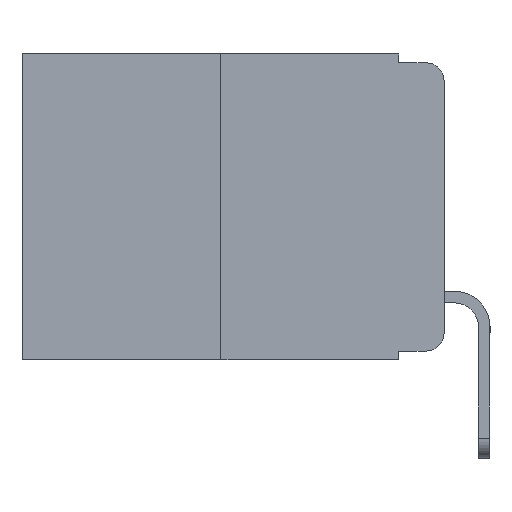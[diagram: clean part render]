
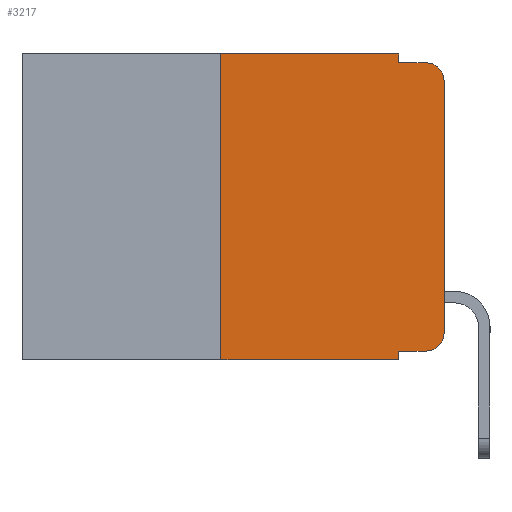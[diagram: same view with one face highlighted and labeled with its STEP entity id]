
A CAD part, left-side view. The second image highlights one B-rep face of the part: STEP entity #3217.
In plain terms, the highlighted planar face has unit normal (-1, 0, 0).
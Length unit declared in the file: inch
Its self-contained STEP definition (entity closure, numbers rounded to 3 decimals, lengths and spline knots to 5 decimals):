
#124 = DIRECTION ( 'NONE',  ( -1., 0., 0. ) ) ;
#164 = EDGE_CURVE ( 'NONE', #3692, #11621, #11876, .T. ) ;
#549 = PLANE ( 'NONE',  #6220 ) ;
#786 = ORIENTED_EDGE ( 'NONE', *, *, #994, .F. ) ;
#886 = EDGE_CURVE ( 'NONE', #7937, #5709, #5619, .T. ) ;
#915 = EDGE_CURVE ( 'NONE', #3985, #5709, #7725, .T. ) ;
#959 = EDGE_CURVE ( 'NONE', #8547, #3692, #6330, .T. ) ;
#992 = EDGE_CURVE ( 'NONE', #2459, #7937, #12639, .T. ) ;
#994 = EDGE_CURVE ( 'NONE', #11621, #3985, #9289, .T. ) ;
#1360 = ORIENTED_EDGE ( 'NONE', *, *, #164, .F. ) ;
#1522 = EDGE_CURVE ( 'NONE', #11440, #16614, #14480, .T. ) ;
#1541 = CARTESIAN_POINT ( 'NONE',  ( 0., 0.02, -0.01 ) ) ;
#2351 = CARTESIAN_POINT ( 'NONE',  ( 0., 0.25, -0.343 ) ) ;
#2446 = ORIENTED_EDGE ( 'NONE', *, *, #14874, .F. ) ;
#2459 = VERTEX_POINT ( 'NONE', #6976 ) ;
#2882 = CARTESIAN_POINT ( 'NONE',  ( 0., 0.051, -0.333 ) ) ;
#2959 = ORIENTED_EDGE ( 'NONE', *, *, #9412, .T. ) ;
#3060 = DIRECTION ( 'NONE',  ( 0., 0., -1. ) ) ;
#3217 = ADVANCED_FACE ( 'NONE', ( #4060 ), #549, .F. ) ;
#3358 = CARTESIAN_POINT ( 'NONE',  ( 0., 0.02, -0.313 ) ) ;
#3692 = VERTEX_POINT ( 'NONE', #15382 ) ;
#3832 = EDGE_CURVE ( 'NONE', #8547, #16906, #17649, .T. ) ;
#3947 = DIRECTION ( 'NONE',  ( 1., 0., 0. ) ) ;
#3985 = VERTEX_POINT ( 'NONE', #11628 ) ;
#4060 = FACE_OUTER_BOUND ( 'NONE', #10998, .T. ) ;
#4124 = AXIS2_PLACEMENT_3D ( 'NONE', #6033, #124, #3060 ) ;
#4198 = VECTOR ( 'NONE', #5405, 39.37008 ) ;
#4660 = ORIENTED_EDGE ( 'NONE', *, *, #915, .F. ) ;
#4742 = VECTOR ( 'NONE', #6989, 39.37008 ) ;
#4897 = DIRECTION ( 'NONE',  ( 0., 0., -1. ) ) ;
#5322 = CARTESIAN_POINT ( 'NONE',  ( 0., 0.051, -0.01 ) ) ;
#5331 = VECTOR ( 'NONE', #10508, 39.37008 ) ;
#5405 = DIRECTION ( 'NONE',  ( 0., -1., 0. ) ) ;
#5424 = CARTESIAN_POINT ( 'NONE',  ( 0., 0., 0. ) ) ;
#5515 = DIRECTION ( 'NONE',  ( 0., 0., 1. ) ) ;
#5593 = ORIENTED_EDGE ( 'NONE', *, *, #959, .F. ) ;
#5619 = CIRCLE ( 'NONE', #4124, 0.02 ) ;
#5709 = VERTEX_POINT ( 'NONE', #1541 ) ;
#6033 = CARTESIAN_POINT ( 'NONE',  ( 0., 0.02, -0.03 ) ) ;
#6220 = AXIS2_PLACEMENT_3D ( 'NONE', #15824, #3947, #13518 ) ;
#6330 = LINE ( 'NONE', #8835, #7257 ) ;
#6976 = CARTESIAN_POINT ( 'NONE',  ( 0., 0., -0.313 ) ) ;
#6989 = DIRECTION ( 'NONE',  ( 0., -1., 0. ) ) ;
#7189 = AXIS2_PLACEMENT_3D ( 'NONE', #3358, #13056, #4897 ) ;
#7226 = VECTOR ( 'NONE', #15899, 39.37008 ) ;
#7257 = VECTOR ( 'NONE', #9005, 39.37008 ) ;
#7295 = CARTESIAN_POINT ( 'NONE',  ( 0., 0.051, -0.333 ) ) ;
#7679 = DIRECTION ( 'NONE',  ( 0., 0., -1. ) ) ;
#7725 = LINE ( 'NONE', #5322, #4198 ) ;
#7937 = VERTEX_POINT ( 'NONE', #15793 ) ;
#8032 = CIRCLE ( 'NONE', #7189, 0.02 ) ;
#8547 = VERTEX_POINT ( 'NONE', #2351 ) ;
#8835 = CARTESIAN_POINT ( 'NONE',  ( 0., 0.25, 0. ) ) ;
#9005 = DIRECTION ( 'NONE',  ( 0., 0., 1. ) ) ;
#9289 = LINE ( 'NONE', #15626, #15413 ) ;
#9412 = EDGE_CURVE ( 'NONE', #16614, #2459, #8032, .T. ) ;
#10404 = CARTESIAN_POINT ( 'NONE',  ( 0., 0.051, 0. ) ) ;
#10508 = DIRECTION ( 'NONE',  ( 0., -1., 0. ) ) ;
#10998 = EDGE_LOOP ( 'NONE', ( #11306, #11693, #4660, #786, #1360, #5593, #16322, #2446, #13564, #2959 ) ) ;
#11306 = ORIENTED_EDGE ( 'NONE', *, *, #992, .T. ) ;
#11440 = VERTEX_POINT ( 'NONE', #2882 ) ;
#11621 = VERTEX_POINT ( 'NONE', #10404 ) ;
#11628 = CARTESIAN_POINT ( 'NONE',  ( 0., 0.051, -0.01 ) ) ;
#11693 = ORIENTED_EDGE ( 'NONE', *, *, #886, .T. ) ;
#11854 = LINE ( 'NONE', #15244, #17735 ) ;
#11876 = LINE ( 'NONE', #14030, #5331 ) ;
#12639 = LINE ( 'NONE', #5424, #13376 ) ;
#13056 = DIRECTION ( 'NONE',  ( -1., 0., 0. ) ) ;
#13376 = VECTOR ( 'NONE', #5515, 39.37008 ) ;
#13446 = CARTESIAN_POINT ( 'NONE',  ( 0., 0.02, -0.333 ) ) ;
#13518 = DIRECTION ( 'NONE',  ( 0., 0., -1. ) ) ;
#13564 = ORIENTED_EDGE ( 'NONE', *, *, #1522, .T. ) ;
#14030 = CARTESIAN_POINT ( 'NONE',  ( 0., 0.473, 0. ) ) ;
#14480 = LINE ( 'NONE', #7295, #7226 ) ;
#14631 = DIRECTION ( 'NONE',  ( 0., 0., -1. ) ) ;
#14704 = CARTESIAN_POINT ( 'NONE',  ( 0., 0.473, -0.343 ) ) ;
#14750 = CARTESIAN_POINT ( 'NONE',  ( 0., 0.051, -0.343 ) ) ;
#14874 = EDGE_CURVE ( 'NONE', #11440, #16906, #11854, .T. ) ;
#15244 = CARTESIAN_POINT ( 'NONE',  ( 0., 0.051, 0. ) ) ;
#15382 = CARTESIAN_POINT ( 'NONE',  ( 0., 0.25, 0. ) ) ;
#15413 = VECTOR ( 'NONE', #14631, 39.37008 ) ;
#15626 = CARTESIAN_POINT ( 'NONE',  ( 0., 0.051, 0. ) ) ;
#15793 = CARTESIAN_POINT ( 'NONE',  ( 0., 0., -0.03 ) ) ;
#15824 = CARTESIAN_POINT ( 'NONE',  ( 0., 0.473, 0. ) ) ;
#15899 = DIRECTION ( 'NONE',  ( 0., -1., 0. ) ) ;
#16322 = ORIENTED_EDGE ( 'NONE', *, *, #3832, .T. ) ;
#16614 = VERTEX_POINT ( 'NONE', #13446 ) ;
#16906 = VERTEX_POINT ( 'NONE', #14750 ) ;
#17649 = LINE ( 'NONE', #14704, #4742 ) ;
#17735 = VECTOR ( 'NONE', #7679, 39.37008 ) ;
